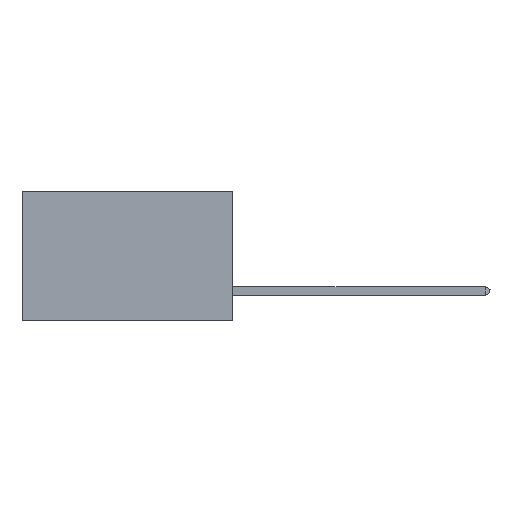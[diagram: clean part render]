
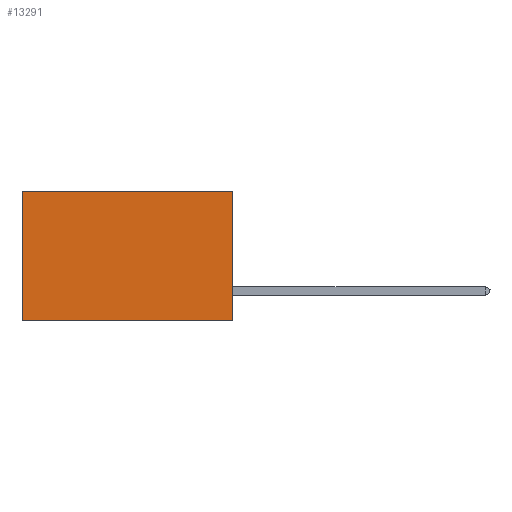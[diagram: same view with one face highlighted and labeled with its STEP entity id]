
A CAD part, left-side view. The second image highlights one B-rep face of the part: STEP entity #13291.
In plain terms, the highlighted planar face has unit normal (-1, 0, 0).
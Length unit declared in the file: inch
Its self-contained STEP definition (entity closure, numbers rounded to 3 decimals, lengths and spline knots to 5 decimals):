
#676 = AXIS2_PLACEMENT_3D ( 'NONE', #18985, #14187, #31304 ) ;
#1283 = CARTESIAN_POINT ( 'NONE',  ( 0.2875, 0., 0. ) ) ;
#4114 = DIRECTION ( 'NONE',  ( 0., 0., -1. ) ) ;
#4126 = LINE ( 'NONE', #12567, #30941 ) ;
#5821 = LINE ( 'NONE', #13871, #13516 ) ;
#6354 = EDGE_CURVE ( 'NONE', #22370, #27000, #4126, .T. ) ;
#6443 = PLANE ( 'NONE',  #676 ) ;
#6782 = EDGE_CURVE ( 'NONE', #7838, #30920, #25546, .T. ) ;
#7588 = ORIENTED_EDGE ( 'NONE', *, *, #6782, .T. ) ;
#7838 = VERTEX_POINT ( 'NONE', #1283 ) ;
#7863 = CARTESIAN_POINT ( 'NONE',  ( 0.2875, 0.6, -0.37 ) ) ;
#10708 = FACE_OUTER_BOUND ( 'NONE', #27688, .T. ) ;
#12567 = CARTESIAN_POINT ( 'NONE',  ( 0.2875, 0., -0.37 ) ) ;
#13291 = ADVANCED_FACE ( 'NONE', ( #10708 ), #6443, .F. ) ;
#13516 = VECTOR ( 'NONE', #4114, 39.37008 ) ;
#13871 = CARTESIAN_POINT ( 'NONE',  ( 0.2875, 0.6, 0. ) ) ;
#14187 = DIRECTION ( 'NONE',  ( 1., 0., 0. ) ) ;
#16467 = VECTOR ( 'NONE', #20056, 39.37008 ) ;
#17485 = ORIENTED_EDGE ( 'NONE', *, *, #17695, .T. ) ;
#17569 = CARTESIAN_POINT ( 'NONE',  ( 0.2875, 0., 0. ) ) ;
#17613 = ORIENTED_EDGE ( 'NONE', *, *, #19730, .F. ) ;
#17695 = EDGE_CURVE ( 'NONE', #30920, #27000, #5821, .T. ) ;
#18985 = CARTESIAN_POINT ( 'NONE',  ( 0.2875, 0., 0. ) ) ;
#19730 = EDGE_CURVE ( 'NONE', #7838, #22370, #31398, .T. ) ;
#20056 = DIRECTION ( 'NONE',  ( 0., 0., -1. ) ) ;
#22370 = VERTEX_POINT ( 'NONE', #27171 ) ;
#24854 = CARTESIAN_POINT ( 'NONE',  ( 0.2875, 0.6, 0. ) ) ;
#25546 = LINE ( 'NONE', #30618, #26323 ) ;
#26323 = VECTOR ( 'NONE', #28073, 39.37008 ) ;
#27000 = VERTEX_POINT ( 'NONE', #7863 ) ;
#27142 = ORIENTED_EDGE ( 'NONE', *, *, #6354, .F. ) ;
#27171 = CARTESIAN_POINT ( 'NONE',  ( 0.2875, 0., -0.37 ) ) ;
#27688 = EDGE_LOOP ( 'NONE', ( #17485, #27142, #17613, #7588 ) ) ;
#28073 = DIRECTION ( 'NONE',  ( 0., 1., 0. ) ) ;
#29689 = DIRECTION ( 'NONE',  ( 0., 1., 0. ) ) ;
#30618 = CARTESIAN_POINT ( 'NONE',  ( 0.2875, 0., 0. ) ) ;
#30920 = VERTEX_POINT ( 'NONE', #24854 ) ;
#30941 = VECTOR ( 'NONE', #29689, 39.37008 ) ;
#31304 = DIRECTION ( 'NONE',  ( 0., 0., -1. ) ) ;
#31398 = LINE ( 'NONE', #17569, #16467 ) ;
